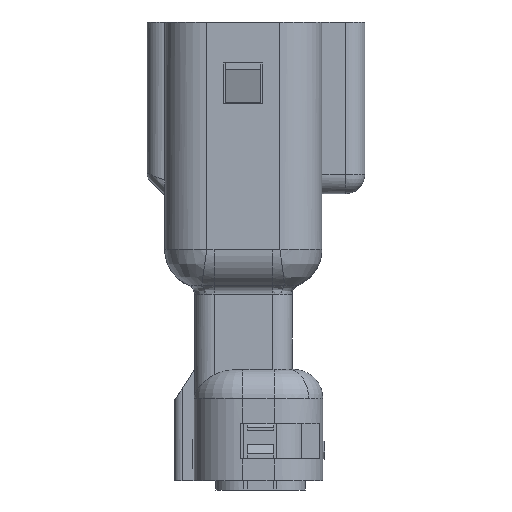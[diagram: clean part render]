
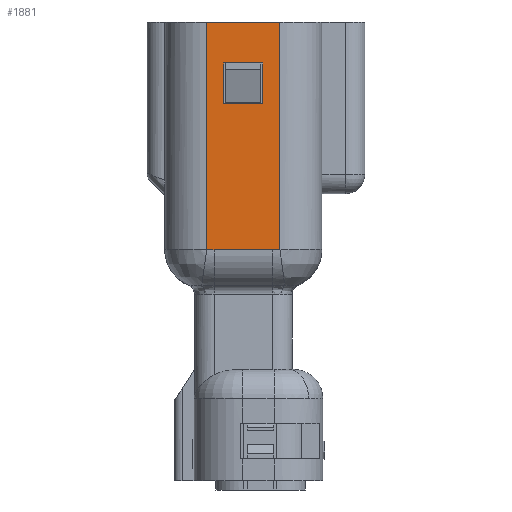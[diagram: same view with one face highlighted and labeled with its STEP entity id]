
A CAD part, left-side view. The second image highlights one B-rep face of the part: STEP entity #1881.
In plain terms, the highlighted face is planar.
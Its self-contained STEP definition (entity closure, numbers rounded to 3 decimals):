
#522 = CARTESIAN_POINT ( 'NONE',  ( 11.7, 5.735, -13.66 ) ) ;
#762 = CARTESIAN_POINT ( 'NONE',  ( 11.7, 5.95, -25.33 ) ) ;
#792 = CARTESIAN_POINT ( 'NONE',  ( 11.7, 2.2, -25.33 ) ) ;
#1098 = CARTESIAN_POINT ( 'NONE',  ( 11.7, 3.075, -21.13 ) ) ;
#1105 = DIRECTION ( 'NONE',  ( 0., 0., -1. ) ) ;
#1539 = AXIS2_PLACEMENT_3D ( 'NONE', #7214, #5048, #29910 ) ;
#1677 = CARTESIAN_POINT ( 'NONE',  ( 11.7, 2.498, -13.654 ) ) ;
#1881 = ADVANCED_FACE ( 'NONE', ( #4879, #30399 ), #15323, .T. ) ;
#2187 = CARTESIAN_POINT ( 'NONE',  ( 11.7, 2.34, -13.668 ) ) ;
#2674 = CARTESIAN_POINT ( 'NONE',  ( 11.7, 5.936, -13.685 ) ) ;
#3159 = EDGE_CURVE ( 'NONE', #26149, #8473, #3240, .T. ) ;
#3240 = LINE ( 'NONE', #762, #14947 ) ;
#3785 = VECTOR ( 'NONE', #19585, 1000. ) ;
#4354 = CARTESIAN_POINT ( 'NONE',  ( 11.7, 2.266, -13.678 ) ) ;
#4703 = CARTESIAN_POINT ( 'NONE',  ( 11.7, 2.2, -13.687 ) ) ;
#4796 = EDGE_CURVE ( 'NONE', #16741, #8473, #30436, .T. ) ;
#4879 = FACE_BOUND ( 'NONE', #28509, .T. ) ;
#5022 = CARTESIAN_POINT ( 'NONE',  ( 11.7, 5.891, -13.679 ) ) ;
#5048 = DIRECTION ( 'NONE',  ( 1., 0., 0. ) ) ;
#6240 = DIRECTION ( 'NONE',  ( 0., 1., 0. ) ) ;
#7194 = EDGE_CURVE ( 'NONE', #16886, #16741, #32196, .T. ) ;
#7214 = CARTESIAN_POINT ( 'NONE',  ( 11.7, 2.2, -25.33 ) ) ;
#8473 = VERTEX_POINT ( 'NONE', #20599 ) ;
#8960 = CARTESIAN_POINT ( 'NONE',  ( 11.7, 3.075, -21.13 ) ) ;
#9624 = EDGE_LOOP ( 'NONE', ( #28178, #26461, #24233, #32274, #27286, #14768 ) ) ;
#9787 = VECTOR ( 'NONE', #13416, 1000. ) ;
#10132 = ORIENTED_EDGE ( 'NONE', *, *, #16427, .T. ) ;
#11226 = LINE ( 'NONE', #11569, #24467 ) ;
#11569 = CARTESIAN_POINT ( 'NONE',  ( 11.7, 3.075, -21.13 ) ) ;
#12158 = VERTEX_POINT ( 'NONE', #13746 ) ;
#12574 = VECTOR ( 'NONE', #29279, 1000. ) ;
#12645 = CARTESIAN_POINT ( 'NONE',  ( 11.7, 5.602, -13.653 ) ) ;
#12796 = CARTESIAN_POINT ( 'NONE',  ( 11.7, 5.818, -13.669 ) ) ;
#13287 = EDGE_CURVE ( 'NONE', #28226, #26149, #17715, .T. ) ;
#13367 = DIRECTION ( 'NONE',  ( 0., 0., 1. ) ) ;
#13416 = DIRECTION ( 'NONE',  ( 0., 0., 1. ) ) ;
#13705 = LINE ( 'NONE', #28753, #20362 ) ;
#13746 = CARTESIAN_POINT ( 'NONE',  ( 11.7, 2.2, -13.687 ) ) ;
#14768 = ORIENTED_EDGE ( 'NONE', *, *, #7194, .F. ) ;
#14800 = CARTESIAN_POINT ( 'NONE',  ( 11.7, 2.421, -13.66 ) ) ;
#14924 = CARTESIAN_POINT ( 'NONE',  ( 11.7, 5.075, -21.13 ) ) ;
#14947 = VECTOR ( 'NONE', #13367, 1000. ) ;
#15130 = CARTESIAN_POINT ( 'NONE',  ( 11.7, 5.95, -13.687 ) ) ;
#15323 = PLANE ( 'NONE',  #1539 ) ;
#15899 = CARTESIAN_POINT ( 'NONE',  ( 11.7, 5.95, -25.33 ) ) ;
#16327 = VERTEX_POINT ( 'NONE', #30799 ) ;
#16427 = EDGE_CURVE ( 'NONE', #31168, #31468, #24139, .T. ) ;
#16741 = VERTEX_POINT ( 'NONE', #22652 ) ;
#16880 = VERTEX_POINT ( 'NONE', #23922 ) ;
#16886 = VERTEX_POINT ( 'NONE', #23770 ) ;
#16955 = CARTESIAN_POINT ( 'NONE',  ( 11.7, 2.549, -13.653 ) ) ;
#17617 = EDGE_CURVE ( 'NONE', #31168, #16880, #11226, .T. ) ;
#17715 = LINE ( 'NONE', #22680, #32530 ) ;
#18230 = DIRECTION ( 'NONE',  ( 0., 0., 1. ) ) ;
#18617 = EDGE_CURVE ( 'NONE', #12158, #16886, #24785, .T. ) ;
#19585 = DIRECTION ( 'NONE',  ( 0., 1., 0. ) ) ;
#20068 = ORIENTED_EDGE ( 'NONE', *, *, #17617, .F. ) ;
#20075 = CARTESIAN_POINT ( 'NONE',  ( 11.7, 2.575, -13.653 ) ) ;
#20362 = VECTOR ( 'NONE', #6240, 1000. ) ;
#20599 = CARTESIAN_POINT ( 'NONE',  ( 11.7, 5.95, -13.687 ) ) ;
#21592 = ORIENTED_EDGE ( 'NONE', *, *, #24841, .F. ) ;
#22652 = CARTESIAN_POINT ( 'NONE',  ( 11.7, 5.575, -13.653 ) ) ;
#22680 = CARTESIAN_POINT ( 'NONE',  ( 11.7, 2.2, -25.33 ) ) ;
#23675 = EDGE_CURVE ( 'NONE', #16880, #16327, #13705, .T. ) ;
#23770 = CARTESIAN_POINT ( 'NONE',  ( 11.7, 2.575, -13.653 ) ) ;
#23922 = CARTESIAN_POINT ( 'NONE',  ( 11.7, 3.075, -23.23 ) ) ;
#24139 = LINE ( 'NONE', #1098, #12574 ) ;
#24233 = ORIENTED_EDGE ( 'NONE', *, *, #13287, .T. ) ;
#24467 = VECTOR ( 'NONE', #1105, 1000. ) ;
#24785 =( BOUNDED_CURVE ( )  B_SPLINE_CURVE ( 3, ( #4703, #29549, #4354, #2187, #14800, #1677, #16955, #32215 ),
 .UNSPECIFIED., .F., .T. ) 
 B_SPLINE_CURVE_WITH_KNOTS ( ( 4, 1, 1, 1, 1, 4 ),
 ( 0., 0.119, 0.327, 0.543, 0.768, 1. ),
 .UNSPECIFIED. ) 
 CURVE ( )  GEOMETRIC_REPRESENTATION_ITEM ( )  RATIONAL_B_SPLINE_CURVE ( ( 1.097, 1.097, 1.097, 1.097, 1.097, 1.097, 1.097, 1.097 ) ) 
 REPRESENTATION_ITEM ( '' )  );
#24841 = EDGE_CURVE ( 'NONE', #16327, #31468, #26151, .T. ) ;
#25988 = CARTESIAN_POINT ( 'NONE',  ( 11.7, 2.2, -25.33 ) ) ;
#26149 = VERTEX_POINT ( 'NONE', #15899 ) ;
#26151 = LINE ( 'NONE', #28487, #9787 ) ;
#26156 = LINE ( 'NONE', #25988, #28365 ) ;
#26164 = EDGE_CURVE ( 'NONE', #28226, #12158, #26156, .T. ) ;
#26461 = ORIENTED_EDGE ( 'NONE', *, *, #26164, .F. ) ;
#27286 = ORIENTED_EDGE ( 'NONE', *, *, #4796, .F. ) ;
#28025 = CARTESIAN_POINT ( 'NONE',  ( 11.7, 5.575, -13.653 ) ) ;
#28178 = ORIENTED_EDGE ( 'NONE', *, *, #18617, .F. ) ;
#28226 = VERTEX_POINT ( 'NONE', #792 ) ;
#28365 = VECTOR ( 'NONE', #18230, 1000. ) ;
#28487 = CARTESIAN_POINT ( 'NONE',  ( 11.7, 5.075, -23.23 ) ) ;
#28509 = EDGE_LOOP ( 'NONE', ( #21592, #28645, #20068, #10132 ) ) ;
#28645 = ORIENTED_EDGE ( 'NONE', *, *, #23675, .F. ) ;
#28753 = CARTESIAN_POINT ( 'NONE',  ( 11.7, 3.075, -23.23 ) ) ;
#29279 = DIRECTION ( 'NONE',  ( 0., 1., 0. ) ) ;
#29549 = CARTESIAN_POINT ( 'NONE',  ( 11.7, 2.218, -13.684 ) ) ;
#29910 = DIRECTION ( 'NONE',  ( 0., 1., 0. ) ) ;
#30399 = FACE_OUTER_BOUND ( 'NONE', #9624, .T. ) ;
#30436 =( BOUNDED_CURVE ( )  B_SPLINE_CURVE ( 3, ( #28025, #12645, #32720, #522, #12796, #5022, #2674, #15130 ),
 .UNSPECIFIED., .F., .T. ) 
 B_SPLINE_CURVE_WITH_KNOTS ( ( 4, 1, 1, 1, 1, 4 ),
 ( 0., 0.24, 0.472, 0.694, 0.908, 1. ),
 .UNSPECIFIED. ) 
 CURVE ( )  GEOMETRIC_REPRESENTATION_ITEM ( )  RATIONAL_B_SPLINE_CURVE ( ( 1.097, 1.097, 1.097, 1.097, 1.097, 1.097, 1.097, 1.097 ) ) 
 REPRESENTATION_ITEM ( '' )  );
#30799 = CARTESIAN_POINT ( 'NONE',  ( 11.7, 5.075, -23.23 ) ) ;
#31168 = VERTEX_POINT ( 'NONE', #8960 ) ;
#31468 = VERTEX_POINT ( 'NONE', #14924 ) ;
#32196 = LINE ( 'NONE', #20075, #3785 ) ;
#32215 = CARTESIAN_POINT ( 'NONE',  ( 11.7, 2.575, -13.653 ) ) ;
#32274 = ORIENTED_EDGE ( 'NONE', *, *, #3159, .T. ) ;
#32530 = VECTOR ( 'NONE', #32813, 1000. ) ;
#32720 = CARTESIAN_POINT ( 'NONE',  ( 11.7, 5.654, -13.654 ) ) ;
#32813 = DIRECTION ( 'NONE',  ( 0., 1., 0. ) ) ;
